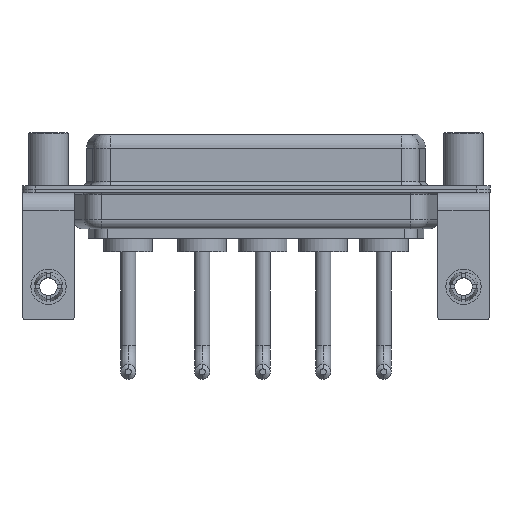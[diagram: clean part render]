
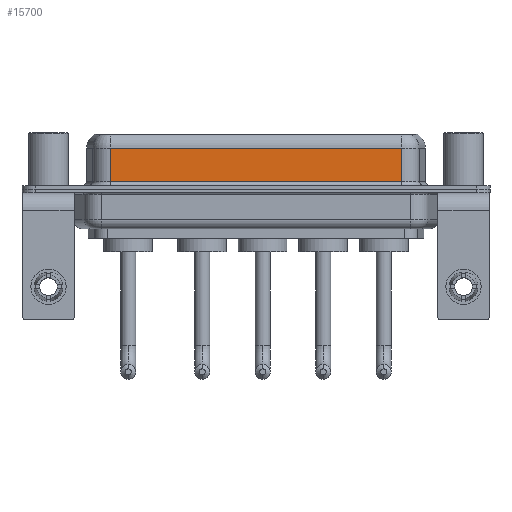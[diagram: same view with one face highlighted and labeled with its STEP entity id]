
A CAD part, front view. The second image highlights one B-rep face of the part: STEP entity #15700.
In plain terms, the highlighted planar face has unit normal (0, -1, 0).
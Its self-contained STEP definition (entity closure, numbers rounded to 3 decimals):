
#654 = VECTOR ( 'NONE', #14225, 1000. ) ;
#1556 = CARTESIAN_POINT ( 'NONE',  ( 40.037, -3.95, 4.65 ) ) ;
#2081 = DIRECTION ( 'NONE',  ( 0., 0., -1. ) ) ;
#2502 = DIRECTION ( 'NONE',  ( 0., 1., 0. ) ) ;
#3353 = LINE ( 'NONE', #6009, #9195 ) ;
#3861 = DIRECTION ( 'NONE',  ( 0., 0., 1. ) ) ;
#3932 = LINE ( 'NONE', #13216, #12994 ) ;
#4027 = ORIENTED_EDGE ( 'NONE', *, *, #15238, .T. ) ;
#4836 = LINE ( 'NONE', #14129, #654 ) ;
#5023 = AXIS2_PLACEMENT_3D ( 'NONE', #13063, #2502, #3861 ) ;
#5046 = CARTESIAN_POINT ( 'NONE',  ( 7.013, -3.95, 0.9 ) ) ;
#5223 = DIRECTION ( 'NONE',  ( 1., 0., 0. ) ) ;
#5788 = EDGE_CURVE ( 'NONE', #11818, #15068, #3932, .T. ) ;
#6009 = CARTESIAN_POINT ( 'NONE',  ( 40.037, -3.95, 6.4 ) ) ;
#6755 = DIRECTION ( 'NONE',  ( -1., 0., 0. ) ) ;
#6856 = ORIENTED_EDGE ( 'NONE', *, *, #5788, .T. ) ;
#7192 = EDGE_CURVE ( 'NONE', #13473, #15068, #3353, .T. ) ;
#7565 = VERTEX_POINT ( 'NONE', #15023 ) ;
#8118 = ORIENTED_EDGE ( 'NONE', *, *, #15941, .T. ) ;
#8782 = CARTESIAN_POINT ( 'NONE',  ( 40.037, -3.95, 4.65 ) ) ;
#8887 = PLANE ( 'NONE',  #5023 ) ;
#9195 = VECTOR ( 'NONE', #2081, 1000. ) ;
#9363 = CARTESIAN_POINT ( 'NONE',  ( 40.037, -3.95, 0.9 ) ) ;
#11818 = VERTEX_POINT ( 'NONE', #5046 ) ;
#12639 = VECTOR ( 'NONE', #6755, 1000. ) ;
#12994 = VECTOR ( 'NONE', #5223, 1000. ) ;
#13063 = CARTESIAN_POINT ( 'NONE',  ( 40.037, -3.95, 6.4 ) ) ;
#13216 = CARTESIAN_POINT ( 'NONE',  ( 40.037, -3.95, 0.9 ) ) ;
#13473 = VERTEX_POINT ( 'NONE', #8782 ) ;
#14129 = CARTESIAN_POINT ( 'NONE',  ( 7.013, -3.95, 6.4 ) ) ;
#14225 = DIRECTION ( 'NONE',  ( 0., 0., -1. ) ) ;
#14317 = ORIENTED_EDGE ( 'NONE', *, *, #7192, .F. ) ;
#14515 = LINE ( 'NONE', #1556, #12639 ) ;
#15023 = CARTESIAN_POINT ( 'NONE',  ( 7.013, -3.95, 4.65 ) ) ;
#15068 = VERTEX_POINT ( 'NONE', #9363 ) ;
#15238 = EDGE_CURVE ( 'NONE', #7565, #11818, #4836, .T. ) ;
#15629 = FACE_OUTER_BOUND ( 'NONE', #16381, .T. ) ;
#15700 = ADVANCED_FACE ( 'NONE', ( #15629 ), #8887, .F. ) ;
#15941 = EDGE_CURVE ( 'NONE', #13473, #7565, #14515, .T. ) ;
#16381 = EDGE_LOOP ( 'NONE', ( #14317, #8118, #4027, #6856 ) ) ;
